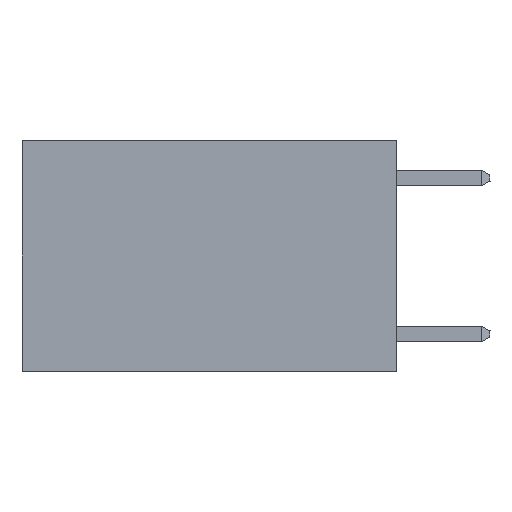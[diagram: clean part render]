
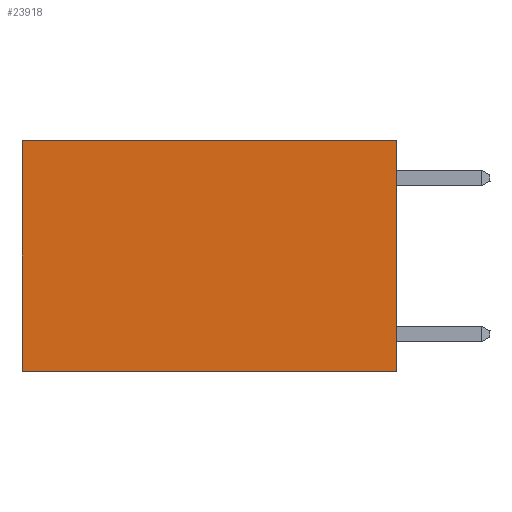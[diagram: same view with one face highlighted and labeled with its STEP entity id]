
A CAD part, left-side view. The second image highlights one B-rep face of the part: STEP entity #23918.
In plain terms, the highlighted planar face has unit normal (-1, 0, 0).
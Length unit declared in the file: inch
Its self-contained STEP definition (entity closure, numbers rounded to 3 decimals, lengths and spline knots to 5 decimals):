
#1695 = LINE ( 'NONE', #8402, #20341 ) ;
#2214 = AXIS2_PLACEMENT_3D ( 'NONE', #5813, #23162, #11802 ) ;
#2945 = FACE_OUTER_BOUND ( 'NONE', #15535, .T. ) ;
#3103 = EDGE_CURVE ( 'NONE', #21700, #24209, #21960, .T. ) ;
#3801 = ORIENTED_EDGE ( 'NONE', *, *, #12312, .T. ) ;
#4747 = DIRECTION ( 'NONE',  ( 0., 1., 0. ) ) ;
#5813 = CARTESIAN_POINT ( 'NONE',  ( 0.2625, 0., 0. ) ) ;
#5944 = LINE ( 'NONE', #17394, #11309 ) ;
#6491 = DIRECTION ( 'NONE',  ( 0., 0., -1. ) ) ;
#6608 = CARTESIAN_POINT ( 'NONE',  ( 0.2625, 0.6, 0. ) ) ;
#8002 = PLANE ( 'NONE',  #2214 ) ;
#8301 = VECTOR ( 'NONE', #16820, 39.37008 ) ;
#8402 = CARTESIAN_POINT ( 'NONE',  ( 0.2625, 0., 0. ) ) ;
#8602 = LINE ( 'NONE', #24336, #8301 ) ;
#9179 = CARTESIAN_POINT ( 'NONE',  ( 0.2625, 0., -0.37 ) ) ;
#9618 = VERTEX_POINT ( 'NONE', #6608 ) ;
#10399 = EDGE_CURVE ( 'NONE', #24209, #23873, #8602, .T. ) ;
#11309 = VECTOR ( 'NONE', #6491, 39.37008 ) ;
#11802 = DIRECTION ( 'NONE',  ( 0., 0., -1. ) ) ;
#12312 = EDGE_CURVE ( 'NONE', #21700, #9618, #1695, .T. ) ;
#13116 = CARTESIAN_POINT ( 'NONE',  ( 0.2625, 0., 0. ) ) ;
#13906 = ORIENTED_EDGE ( 'NONE', *, *, #10399, .F. ) ;
#14837 = DIRECTION ( 'NONE',  ( 0., 0., -1. ) ) ;
#15535 = EDGE_LOOP ( 'NONE', ( #16993, #13906, #17000, #3801 ) ) ;
#16820 = DIRECTION ( 'NONE',  ( 0., 1., 0. ) ) ;
#16993 = ORIENTED_EDGE ( 'NONE', *, *, #23587, .T. ) ;
#17000 = ORIENTED_EDGE ( 'NONE', *, *, #3103, .F. ) ;
#17394 = CARTESIAN_POINT ( 'NONE',  ( 0.2625, 0.6, 0. ) ) ;
#19034 = CARTESIAN_POINT ( 'NONE',  ( 0.2625, 0.6, -0.37 ) ) ;
#20341 = VECTOR ( 'NONE', #4747, 39.37008 ) ;
#21700 = VERTEX_POINT ( 'NONE', #23870 ) ;
#21960 = LINE ( 'NONE', #13116, #23454 ) ;
#23162 = DIRECTION ( 'NONE',  ( 1., 0., 0. ) ) ;
#23454 = VECTOR ( 'NONE', #14837, 39.37008 ) ;
#23587 = EDGE_CURVE ( 'NONE', #9618, #23873, #5944, .T. ) ;
#23870 = CARTESIAN_POINT ( 'NONE',  ( 0.2625, 0., 0. ) ) ;
#23873 = VERTEX_POINT ( 'NONE', #19034 ) ;
#23918 = ADVANCED_FACE ( 'NONE', ( #2945 ), #8002, .F. ) ;
#24209 = VERTEX_POINT ( 'NONE', #9179 ) ;
#24336 = CARTESIAN_POINT ( 'NONE',  ( 0.2625, 0., -0.37 ) ) ;
